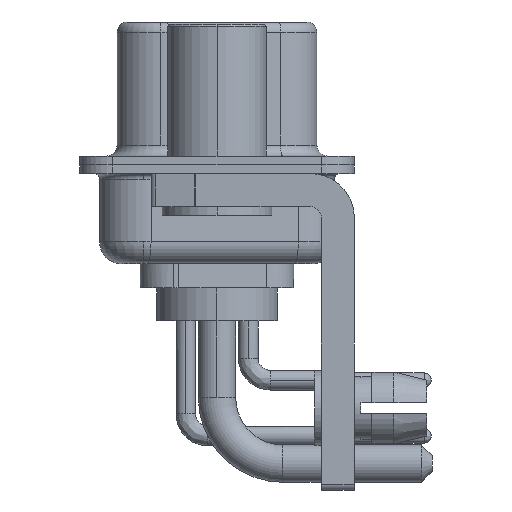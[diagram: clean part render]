
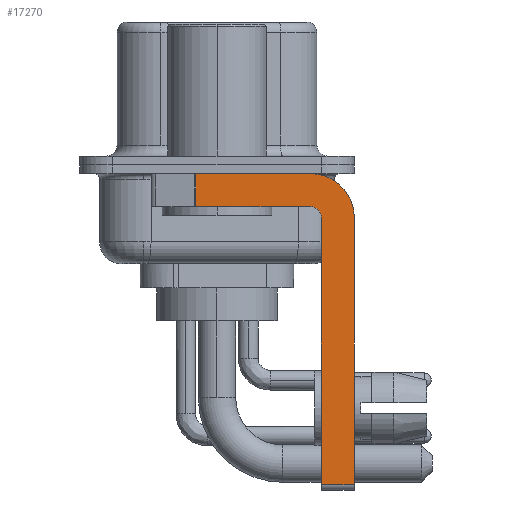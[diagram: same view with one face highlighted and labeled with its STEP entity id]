
A CAD part, left-side view. The second image highlights one B-rep face of the part: STEP entity #17270.
In plain terms, the highlighted planar face has unit normal (-1, 0, 0).
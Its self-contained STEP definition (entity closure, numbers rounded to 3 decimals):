
#364 = ORIENTED_EDGE ( 'NONE', *, *, #2957, .T. ) ;
#578 = LINE ( 'NONE', #10992, #25585 ) ;
#896 = ORIENTED_EDGE ( 'NONE', *, *, #24722, .F. ) ;
#903 = DIRECTION ( 'NONE',  ( 1., 0., 0. ) ) ;
#1133 = EDGE_CURVE ( 'NONE', #19979, #16556, #22987, .T. ) ;
#2080 = CARTESIAN_POINT ( 'NONE',  ( -2.9, -4.75, -14.55 ) ) ;
#2397 = DIRECTION ( 'NONE',  ( 0., 0., 1. ) ) ;
#2957 = EDGE_CURVE ( 'NONE', #6870, #17399, #5131, .T. ) ;
#4022 = LINE ( 'NONE', #14576, #18829 ) ;
#4133 = CARTESIAN_POINT ( 'NONE',  ( -2.9, -6.25, -2.4 ) ) ;
#5131 = LINE ( 'NONE', #7185, #25546 ) ;
#5314 = CARTESIAN_POINT ( 'NONE',  ( -2.9, -4.25, -0.4 ) ) ;
#6544 = AXIS2_PLACEMENT_3D ( 'NONE', #26431, #27096, #2397 ) ;
#6596 = VERTEX_POINT ( 'NONE', #10575 ) ;
#6870 = VERTEX_POINT ( 'NONE', #8912 ) ;
#7185 = CARTESIAN_POINT ( 'NONE',  ( -2.9, 0.978, -1.9 ) ) ;
#7207 = DIRECTION ( 'NONE',  ( 0., -1., 0. ) ) ;
#7495 = PLANE ( 'NONE',  #24239 ) ;
#7901 = CIRCLE ( 'NONE', #26728, 2. ) ;
#8175 = DIRECTION ( 'NONE',  ( 0., 0., 1. ) ) ;
#8682 = DIRECTION ( 'NONE',  ( 0., 0., -1. ) ) ;
#8743 = CIRCLE ( 'NONE', #6544, 0.5 ) ;
#8912 = CARTESIAN_POINT ( 'NONE',  ( -2.9, 0.978, -0.4 ) ) ;
#9315 = CARTESIAN_POINT ( 'NONE',  ( -2.9, -4.75, -2.4 ) ) ;
#9428 = FACE_OUTER_BOUND ( 'NONE', #17218, .T. ) ;
#9845 = ORIENTED_EDGE ( 'NONE', *, *, #18869, .F. ) ;
#10575 = CARTESIAN_POINT ( 'NONE',  ( -2.9, -4.25, -1.9 ) ) ;
#10732 = CARTESIAN_POINT ( 'NONE',  ( -2.9, -4.25, -2.4 ) ) ;
#10992 = CARTESIAN_POINT ( 'NONE',  ( -2.9, -4.25, -1.9 ) ) ;
#11548 = ORIENTED_EDGE ( 'NONE', *, *, #1133, .T. ) ;
#11752 = CARTESIAN_POINT ( 'NONE',  ( -2.9, -6.25, -14.55 ) ) ;
#12512 = DIRECTION ( 'NONE',  ( 0., -1., 0. ) ) ;
#13581 = EDGE_CURVE ( 'NONE', #21625, #6596, #8743, .T. ) ;
#13611 = VECTOR ( 'NONE', #8175, 1000. ) ;
#14406 = DIRECTION ( 'NONE',  ( 0., 0., -1. ) ) ;
#14576 = CARTESIAN_POINT ( 'NONE',  ( -2.9, 3., -0.4 ) ) ;
#14592 = VECTOR ( 'NONE', #7207, 1000. ) ;
#14609 = CARTESIAN_POINT ( 'NONE',  ( -2.9, -6.25, -2.4 ) ) ;
#16556 = VERTEX_POINT ( 'NONE', #11752 ) ;
#16603 = LINE ( 'NONE', #4133, #22048 ) ;
#17218 = EDGE_LOOP ( 'NONE', ( #21524, #364, #23125, #17404, #896, #11548, #9845, #20799 ) ) ;
#17270 = ADVANCED_FACE ( 'NONE', ( #9428 ), #7495, .F. ) ;
#17399 = VERTEX_POINT ( 'NONE', #18452 ) ;
#17404 = ORIENTED_EDGE ( 'NONE', *, *, #13581, .F. ) ;
#17444 = DIRECTION ( 'NONE',  ( 0., 1., 0. ) ) ;
#18452 = CARTESIAN_POINT ( 'NONE',  ( -2.9, 0.978, -1.9 ) ) ;
#18626 = EDGE_CURVE ( 'NONE', #6596, #17399, #578, .T. ) ;
#18829 = VECTOR ( 'NONE', #12512, 1000. ) ;
#18869 = EDGE_CURVE ( 'NONE', #24710, #16556, #16603, .T. ) ;
#19093 = DIRECTION ( 'NONE',  ( 1., 0., 0. ) ) ;
#19979 = VERTEX_POINT ( 'NONE', #2080 ) ;
#20799 = ORIENTED_EDGE ( 'NONE', *, *, #24351, .F. ) ;
#21462 = CARTESIAN_POINT ( 'NONE',  ( -2.9, -4.25, -14.55 ) ) ;
#21488 = CARTESIAN_POINT ( 'NONE',  ( -2.9, -4.25, -2.4 ) ) ;
#21524 = ORIENTED_EDGE ( 'NONE', *, *, #24167, .F. ) ;
#21625 = VERTEX_POINT ( 'NONE', #9315 ) ;
#22048 = VECTOR ( 'NONE', #14406, 1000. ) ;
#22971 = LINE ( 'NONE', #26813, #13611 ) ;
#22987 = LINE ( 'NONE', #21462, #14592 ) ;
#23125 = ORIENTED_EDGE ( 'NONE', *, *, #18626, .F. ) ;
#23580 = VERTEX_POINT ( 'NONE', #5314 ) ;
#24084 = DIRECTION ( 'NONE',  ( 0., 0., -1. ) ) ;
#24167 = EDGE_CURVE ( 'NONE', #6870, #23580, #4022, .T. ) ;
#24239 = AXIS2_PLACEMENT_3D ( 'NONE', #21488, #903, #24084 ) ;
#24351 = EDGE_CURVE ( 'NONE', #23580, #24710, #7901, .T. ) ;
#24710 = VERTEX_POINT ( 'NONE', #14609 ) ;
#24722 = EDGE_CURVE ( 'NONE', #19979, #21625, #22971, .T. ) ;
#25546 = VECTOR ( 'NONE', #26234, 1000. ) ;
#25585 = VECTOR ( 'NONE', #17444, 1000. ) ;
#26234 = DIRECTION ( 'NONE',  ( 0., 0., -1. ) ) ;
#26431 = CARTESIAN_POINT ( 'NONE',  ( -2.9, -4.25, -2.4 ) ) ;
#26728 = AXIS2_PLACEMENT_3D ( 'NONE', #10732, #19093, #8682 ) ;
#26813 = CARTESIAN_POINT ( 'NONE',  ( -2.9, -4.75, -14.8 ) ) ;
#27096 = DIRECTION ( 'NONE',  ( -1., 0., 0. ) ) ;
